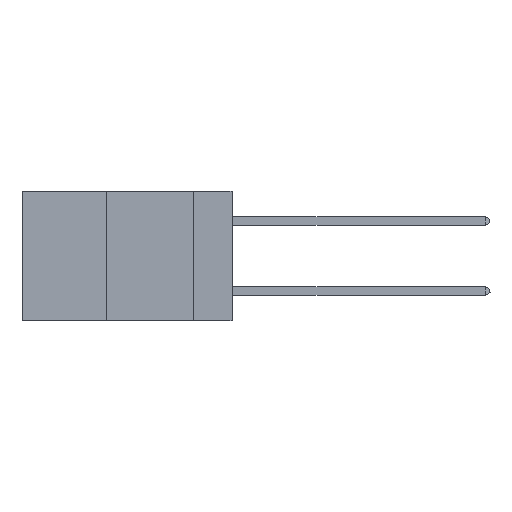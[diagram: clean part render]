
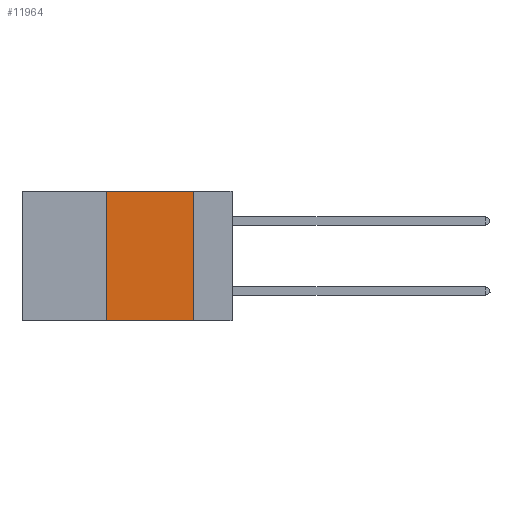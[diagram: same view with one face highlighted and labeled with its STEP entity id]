
A CAD part, left-side view. The second image highlights one B-rep face of the part: STEP entity #11964.
In plain terms, the highlighted planar face has unit normal (-1, 0, 0).
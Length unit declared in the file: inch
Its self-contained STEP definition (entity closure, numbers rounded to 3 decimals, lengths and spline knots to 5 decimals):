
#470 = AXIS2_PLACEMENT_3D ( 'NONE', #10454, #35106, #14195 ) ;
#5054 = EDGE_CURVE ( 'NONE', #9691, #41723, #15935, .T. ) ;
#6028 = VECTOR ( 'NONE', #40349, 39.37008 ) ;
#6715 = ORIENTED_EDGE ( 'NONE', *, *, #19716, .F. ) ;
#6911 = CARTESIAN_POINT ( 'NONE',  ( 0., 0.11, 0. ) ) ;
#8687 = CARTESIAN_POINT ( 'NONE',  ( 0., 0.11, 0. ) ) ;
#9592 = VERTEX_POINT ( 'NONE', #24110 ) ;
#9691 = VERTEX_POINT ( 'NONE', #41294 ) ;
#10454 = CARTESIAN_POINT ( 'NONE',  ( 0., 0.6, 0. ) ) ;
#10904 = VECTOR ( 'NONE', #19520, 39.37008 ) ;
#11964 = ADVANCED_FACE ( 'NONE', ( #13931 ), #31703, .F. ) ;
#12436 = DIRECTION ( 'NONE',  ( 0., 0., -1. ) ) ;
#12875 = EDGE_CURVE ( 'NONE', #9592, #9691, #38693, .T. ) ;
#13931 = FACE_OUTER_BOUND ( 'NONE', #14635, .T. ) ;
#14195 = DIRECTION ( 'NONE',  ( 0., 0., -1. ) ) ;
#14314 = EDGE_CURVE ( 'NONE', #9592, #24100, #38577, .T. ) ;
#14339 = LINE ( 'NONE', #8687, #26184 ) ;
#14635 = EDGE_LOOP ( 'NONE', ( #6715, #20482, #43892, #31240 ) ) ;
#15935 = LINE ( 'NONE', #30322, #6028 ) ;
#19520 = DIRECTION ( 'NONE',  ( 0., 0., 1. ) ) ;
#19716 = EDGE_CURVE ( 'NONE', #41723, #24100, #14339, .T. ) ;
#20482 = ORIENTED_EDGE ( 'NONE', *, *, #5054, .F. ) ;
#21563 = VECTOR ( 'NONE', #43335, 39.37008 ) ;
#24100 = VERTEX_POINT ( 'NONE', #25958 ) ;
#24110 = CARTESIAN_POINT ( 'NONE',  ( 0., 0.36, -0.37 ) ) ;
#25958 = CARTESIAN_POINT ( 'NONE',  ( 0., 0.11, -0.37 ) ) ;
#26184 = VECTOR ( 'NONE', #12436, 39.37008 ) ;
#30322 = CARTESIAN_POINT ( 'NONE',  ( 0., 0.6, 0. ) ) ;
#31240 = ORIENTED_EDGE ( 'NONE', *, *, #14314, .T. ) ;
#31703 = PLANE ( 'NONE',  #470 ) ;
#35106 = DIRECTION ( 'NONE',  ( 1., 0., 0. ) ) ;
#36647 = CARTESIAN_POINT ( 'NONE',  ( 0., 0.36, 0. ) ) ;
#38577 = LINE ( 'NONE', #39994, #21563 ) ;
#38693 = LINE ( 'NONE', #36647, #10904 ) ;
#39994 = CARTESIAN_POINT ( 'NONE',  ( 0., 0.6, -0.37 ) ) ;
#40349 = DIRECTION ( 'NONE',  ( 0., -1., 0. ) ) ;
#41294 = CARTESIAN_POINT ( 'NONE',  ( 0., 0.36, 0. ) ) ;
#41723 = VERTEX_POINT ( 'NONE', #6911 ) ;
#43335 = DIRECTION ( 'NONE',  ( 0., -1., 0. ) ) ;
#43892 = ORIENTED_EDGE ( 'NONE', *, *, #12875, .F. ) ;
